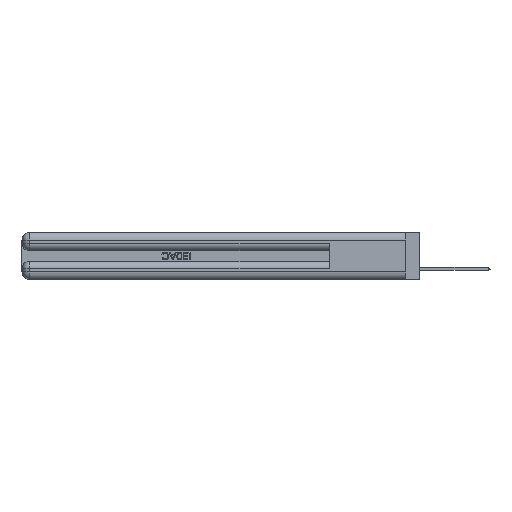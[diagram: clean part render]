
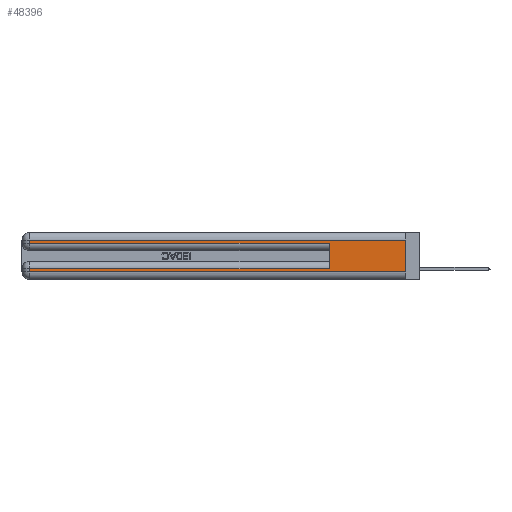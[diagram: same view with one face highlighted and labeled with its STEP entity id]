
A CAD part, left-side view. The second image highlights one B-rep face of the part: STEP entity #48396.
In plain terms, the highlighted planar face has unit normal (-1, 0, 0).
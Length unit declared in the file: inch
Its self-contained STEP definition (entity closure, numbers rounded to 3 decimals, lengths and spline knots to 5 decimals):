
#405 = DIRECTION ( 'NONE',  ( 0., 1., 0. ) ) ;
#673 = CARTESIAN_POINT ( 'NONE',  ( 0., 0., 0.06 ) ) ;
#1915 = CARTESIAN_POINT ( 'NONE',  ( 0., 2.94, 0.285 ) ) ;
#2739 = VERTEX_POINT ( 'NONE', #8942 ) ;
#3091 = CARTESIAN_POINT ( 'NONE',  ( 0., 2.94, 0.31 ) ) ;
#3826 = EDGE_CURVE ( 'NONE', #13576, #22187, #46297, .T. ) ;
#4170 = EDGE_LOOP ( 'NONE', ( #52042, #49506, #12875, #19583, #42117, #42382, #39500, #20913 ) ) ;
#4790 = DIRECTION ( 'NONE',  ( 0., 0., -1. ) ) ;
#5074 = VECTOR ( 'NONE', #8594, 39.37008 ) ;
#5420 = EDGE_CURVE ( 'NONE', #13576, #11813, #30200, .T. ) ;
#5716 = CARTESIAN_POINT ( 'NONE',  ( 0., 0.6, 0.145 ) ) ;
#6245 = DIRECTION ( 'NONE',  ( 0., 0., -1. ) ) ;
#6282 = CARTESIAN_POINT ( 'NONE',  ( 0., 2.94, 0.37 ) ) ;
#7563 = EDGE_CURVE ( 'NONE', #19535, #20030, #39488, .T. ) ;
#7927 = VECTOR ( 'NONE', #6245, 39.37008 ) ;
#8594 = DIRECTION ( 'NONE',  ( 0., 0., -1. ) ) ;
#8942 = CARTESIAN_POINT ( 'NONE',  ( 0., 0.6, 0.085 ) ) ;
#11373 = CARTESIAN_POINT ( 'NONE',  ( 0., 2.94, 0.06 ) ) ;
#11813 = VERTEX_POINT ( 'NONE', #3091 ) ;
#12680 = CARTESIAN_POINT ( 'NONE',  ( 0., 0.6, 0.285 ) ) ;
#12875 = ORIENTED_EDGE ( 'NONE', *, *, #40076, .T. ) ;
#13576 = VERTEX_POINT ( 'NONE', #33800 ) ;
#13698 = EDGE_CURVE ( 'NONE', #24758, #29768, #43193, .T. ) ;
#14760 = LINE ( 'NONE', #39040, #38836 ) ;
#16202 = LINE ( 'NONE', #5716, #20597 ) ;
#16472 = DIRECTION ( 'NONE',  ( 1., 0., 0. ) ) ;
#17290 = VECTOR ( 'NONE', #32416, 39.37008 ) ;
#19535 = VERTEX_POINT ( 'NONE', #47655 ) ;
#19583 = ORIENTED_EDGE ( 'NONE', *, *, #13698, .T. ) ;
#19703 = CARTESIAN_POINT ( 'NONE',  ( 0., 0., 0.31 ) ) ;
#20030 = VERTEX_POINT ( 'NONE', #11373 ) ;
#20597 = VECTOR ( 'NONE', #46635, 39.37008 ) ;
#20913 = ORIENTED_EDGE ( 'NONE', *, *, #34790, .T. ) ;
#22187 = VERTEX_POINT ( 'NONE', #40373 ) ;
#24758 = VERTEX_POINT ( 'NONE', #1915 ) ;
#25370 = CARTESIAN_POINT ( 'NONE',  ( 0., 0., 0.285 ) ) ;
#26779 = LINE ( 'NONE', #673, #17290 ) ;
#27162 = AXIS2_PLACEMENT_3D ( 'NONE', #40933, #16472, #4790 ) ;
#28013 = VECTOR ( 'NONE', #39198, 39.37008 ) ;
#29768 = VERTEX_POINT ( 'NONE', #12680 ) ;
#29813 = DIRECTION ( 'NONE',  ( 0., -1., 0. ) ) ;
#30200 = LINE ( 'NONE', #19703, #43039 ) ;
#32416 = DIRECTION ( 'NONE',  ( 0., -1., 0. ) ) ;
#33235 = PLANE ( 'NONE',  #27162 ) ;
#33800 = CARTESIAN_POINT ( 'NONE',  ( 0., 0., 0.31 ) ) ;
#34790 = EDGE_CURVE ( 'NONE', #20030, #22187, #26779, .T. ) ;
#37138 = CARTESIAN_POINT ( 'NONE',  ( 0., 0., 0.37 ) ) ;
#38836 = VECTOR ( 'NONE', #405, 39.37008 ) ;
#39040 = CARTESIAN_POINT ( 'NONE',  ( 0., 0., 0.085 ) ) ;
#39198 = DIRECTION ( 'NONE',  ( 0., 0., -1. ) ) ;
#39488 = LINE ( 'NONE', #6282, #28013 ) ;
#39500 = ORIENTED_EDGE ( 'NONE', *, *, #7563, .T. ) ;
#40076 = EDGE_CURVE ( 'NONE', #11813, #24758, #45930, .T. ) ;
#40373 = CARTESIAN_POINT ( 'NONE',  ( 0., 0., 0.06 ) ) ;
#40933 = CARTESIAN_POINT ( 'NONE',  ( 0., 0., 0.37 ) ) ;
#41504 = EDGE_CURVE ( 'NONE', #2739, #19535, #14760, .T. ) ;
#42117 = ORIENTED_EDGE ( 'NONE', *, *, #45065, .F. ) ;
#42382 = ORIENTED_EDGE ( 'NONE', *, *, #41504, .T. ) ;
#43039 = VECTOR ( 'NONE', #47888, 39.37008 ) ;
#43193 = LINE ( 'NONE', #25370, #44402 ) ;
#43675 = FACE_OUTER_BOUND ( 'NONE', #4170, .T. ) ;
#44402 = VECTOR ( 'NONE', #29813, 39.37008 ) ;
#45065 = EDGE_CURVE ( 'NONE', #2739, #29768, #16202, .T. ) ;
#45930 = LINE ( 'NONE', #46404, #7927 ) ;
#46297 = LINE ( 'NONE', #37138, #5074 ) ;
#46404 = CARTESIAN_POINT ( 'NONE',  ( 0., 2.94, 0.37 ) ) ;
#46635 = DIRECTION ( 'NONE',  ( 0., 0., 1. ) ) ;
#47655 = CARTESIAN_POINT ( 'NONE',  ( 0., 2.94, 0.085 ) ) ;
#47888 = DIRECTION ( 'NONE',  ( 0., 1., 0. ) ) ;
#48396 = ADVANCED_FACE ( 'NONE', ( #43675 ), #33235, .F. ) ;
#49506 = ORIENTED_EDGE ( 'NONE', *, *, #5420, .T. ) ;
#52042 = ORIENTED_EDGE ( 'NONE', *, *, #3826, .F. ) ;
